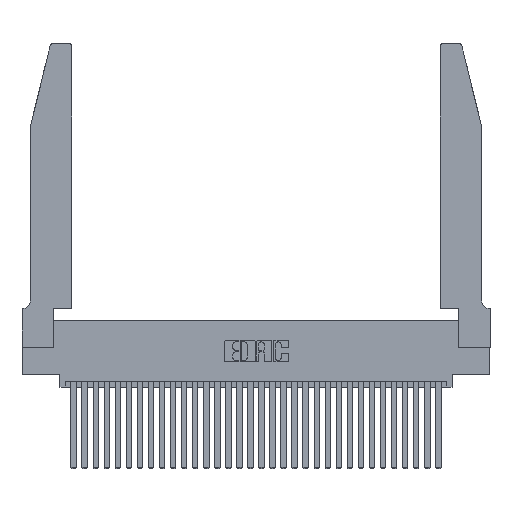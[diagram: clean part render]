
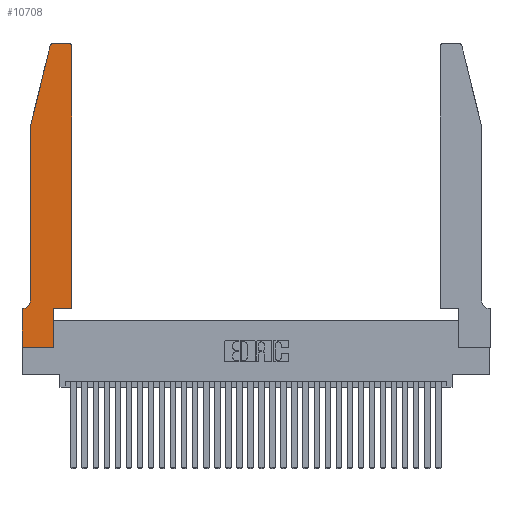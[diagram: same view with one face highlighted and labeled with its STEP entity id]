
A CAD part, top view. The second image highlights one B-rep face of the part: STEP entity #10708.
In plain terms, the highlighted planar face has unit normal (0, 0, 1).
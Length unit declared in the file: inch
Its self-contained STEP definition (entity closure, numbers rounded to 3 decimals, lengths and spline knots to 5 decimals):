
#958 = EDGE_CURVE ( 'NONE', #2977, #4452, #2558, .T. ) ;
#1462 = CARTESIAN_POINT ( 'NONE',  ( 0., 0., 0.37 ) ) ;
#1644 = CARTESIAN_POINT ( 'NONE',  ( 0.284, 2.75, 0.37 ) ) ;
#2005 = CARTESIAN_POINT ( 'NONE',  ( 0.0055, 0.42, 0.37 ) ) ;
#2331 = EDGE_CURVE ( 'NONE', #12128, #19467, #25358, .T. ) ;
#2558 = CIRCLE ( 'NONE', #5105, 0.03 ) ;
#2598 = ORIENTED_EDGE ( 'NONE', *, *, #28789, .T. ) ;
#2977 = VERTEX_POINT ( 'NONE', #1644 ) ;
#3262 = CARTESIAN_POINT ( 'NONE',  ( 0.25487, 2.72718, 0.37 ) ) ;
#3462 = DIRECTION ( 'NONE',  ( 0., 1., 0. ) ) ;
#3615 = CARTESIAN_POINT ( 'NONE',  ( 0.4205, 2.75, 0.37 ) ) ;
#4070 = LINE ( 'NONE', #9349, #22545 ) ;
#4452 = VERTEX_POINT ( 'NONE', #3262 ) ;
#4640 = DIRECTION ( 'NONE',  ( -1., 0., 0. ) ) ;
#5011 = EDGE_LOOP ( 'NONE', ( #26423, #30237, #30179, #9703, #2598, #25439, #15466, #19028, #8001, #28906, #23897, #11461 ) ) ;
#5105 = AXIS2_PLACEMENT_3D ( 'NONE', #8867, #8754, #18470 ) ;
#5704 = DIRECTION ( 'NONE',  ( -0.239, -0.971, 0. ) ) ;
#6570 = CARTESIAN_POINT ( 'NONE',  ( 0.4505, 0.35, 0.37 ) ) ;
#6657 = CARTESIAN_POINT ( 'NONE',  ( 0., 0., 0.37 ) ) ;
#7114 = CARTESIAN_POINT ( 'NONE',  ( 0.4205, 2.72, 0.37 ) ) ;
#7984 = CARTESIAN_POINT ( 'NONE',  ( 0.4505, 0.35, 0.37 ) ) ;
#8001 = ORIENTED_EDGE ( 'NONE', *, *, #20111, .T. ) ;
#8124 = VECTOR ( 'NONE', #22843, 39.37008 ) ;
#8686 = CARTESIAN_POINT ( 'NONE',  ( 0.2865, 0., 0.37 ) ) ;
#8754 = DIRECTION ( 'NONE',  ( 0., 0., 1. ) ) ;
#8867 = CARTESIAN_POINT ( 'NONE',  ( 0.284, 2.72, 0.37 ) ) ;
#8993 = DIRECTION ( 'NONE',  ( 0., 0., 1. ) ) ;
#9085 = LINE ( 'NONE', #15919, #20878 ) ;
#9349 = CARTESIAN_POINT ( 'NONE',  ( 0.0755, 2., 0.37 ) ) ;
#9658 = DIRECTION ( 'NONE',  ( 1., 0., 0. ) ) ;
#9703 = ORIENTED_EDGE ( 'NONE', *, *, #13837, .T. ) ;
#9806 = DIRECTION ( 'NONE',  ( -1., 0., 0. ) ) ;
#9811 = EDGE_CURVE ( 'NONE', #4452, #14387, #9085, .T. ) ;
#9853 = VERTEX_POINT ( 'NONE', #16025 ) ;
#10679 = EDGE_CURVE ( 'NONE', #9853, #25206, #17339, .T. ) ;
#10708 = ADVANCED_FACE ( 'NONE', ( #22335 ), #28796, .T. ) ;
#11073 = CIRCLE ( 'NONE', #18009, 0.07 ) ;
#11461 = ORIENTED_EDGE ( 'NONE', *, *, #2331, .T. ) ;
#11489 = LINE ( 'NONE', #24695, #30460 ) ;
#11821 = EDGE_CURVE ( 'NONE', #19267, #12128, #19568, .T. ) ;
#11926 = CARTESIAN_POINT ( 'NONE',  ( 0., 0.35, 0.37 ) ) ;
#12128 = VERTEX_POINT ( 'NONE', #15202 ) ;
#12404 = CARTESIAN_POINT ( 'NONE',  ( 0.2605, 2.75, 0.37 ) ) ;
#12833 = AXIS2_PLACEMENT_3D ( 'NONE', #7114, #24608, #9658 ) ;
#13027 = LINE ( 'NONE', #1462, #25416 ) ;
#13837 = EDGE_CURVE ( 'NONE', #14387, #19399, #4070, .T. ) ;
#14002 = DIRECTION ( 'NONE',  ( -1., 0., 0. ) ) ;
#14350 = EDGE_CURVE ( 'NONE', #19467, #2977, #30959, .T. ) ;
#14387 = VERTEX_POINT ( 'NONE', #22372 ) ;
#15202 = CARTESIAN_POINT ( 'NONE',  ( 0.4505, 2.72, 0.37 ) ) ;
#15466 = ORIENTED_EDGE ( 'NONE', *, *, #21263, .T. ) ;
#15919 = CARTESIAN_POINT ( 'NONE',  ( 0.0755, 2., 0.37 ) ) ;
#16025 = CARTESIAN_POINT ( 'NONE',  ( 0.0055, 0.35, 0.37 ) ) ;
#16575 = VECTOR ( 'NONE', #14002, 39.37008 ) ;
#16862 = DIRECTION ( 'NONE',  ( 1., 0., 0. ) ) ;
#17339 = LINE ( 'NONE', #21385, #16575 ) ;
#17900 = CARTESIAN_POINT ( 'NONE',  ( 0.4505, 0.35, 0.37 ) ) ;
#18009 = AXIS2_PLACEMENT_3D ( 'NONE', #2005, #19764, #4640 ) ;
#18324 = VECTOR ( 'NONE', #3462, 39.37008 ) ;
#18470 = DIRECTION ( 'NONE',  ( 1., 0., 0. ) ) ;
#19028 = ORIENTED_EDGE ( 'NONE', *, *, #22811, .T. ) ;
#19112 = AXIS2_PLACEMENT_3D ( 'NONE', #21492, #8993, #26432 ) ;
#19267 = VERTEX_POINT ( 'NONE', #7984 ) ;
#19399 = VERTEX_POINT ( 'NONE', #30832 ) ;
#19467 = VERTEX_POINT ( 'NONE', #3615 ) ;
#19568 = LINE ( 'NONE', #6570, #20357 ) ;
#19764 = DIRECTION ( 'NONE',  ( 0., 0., -1. ) ) ;
#20111 = EDGE_CURVE ( 'NONE', #25022, #28366, #24852, .T. ) ;
#20357 = VECTOR ( 'NONE', #24076, 39.37008 ) ;
#20878 = VECTOR ( 'NONE', #5704, 39.37008 ) ;
#21263 = EDGE_CURVE ( 'NONE', #25206, #32402, #11489, .T. ) ;
#21385 = CARTESIAN_POINT ( 'NONE',  ( 0.0755, 0.35, 0.37 ) ) ;
#21492 = CARTESIAN_POINT ( 'NONE',  ( 0., 0.35, 0.37 ) ) ;
#22246 = LINE ( 'NONE', #17900, #8124 ) ;
#22335 = FACE_OUTER_BOUND ( 'NONE', #5011, .T. ) ;
#22372 = CARTESIAN_POINT ( 'NONE',  ( 0.0755, 2., 0.37 ) ) ;
#22545 = VECTOR ( 'NONE', #24403, 39.37008 ) ;
#22811 = EDGE_CURVE ( 'NONE', #32402, #25022, #13027, .T. ) ;
#22843 = DIRECTION ( 'NONE',  ( 1., 0., 0. ) ) ;
#23658 = VECTOR ( 'NONE', #9806, 39.37008 ) ;
#23897 = ORIENTED_EDGE ( 'NONE', *, *, #11821, .T. ) ;
#24076 = DIRECTION ( 'NONE',  ( 0., 1., 0. ) ) ;
#24136 = EDGE_CURVE ( 'NONE', #28366, #19267, #22246, .T. ) ;
#24403 = DIRECTION ( 'NONE',  ( 0., -1., 0. ) ) ;
#24608 = DIRECTION ( 'NONE',  ( 0., 0., 1. ) ) ;
#24695 = CARTESIAN_POINT ( 'NONE',  ( 0., 0., 0.37 ) ) ;
#24852 = LINE ( 'NONE', #25975, #18324 ) ;
#25022 = VERTEX_POINT ( 'NONE', #8686 ) ;
#25206 = VERTEX_POINT ( 'NONE', #11926 ) ;
#25358 = CIRCLE ( 'NONE', #12833, 0.03 ) ;
#25365 = CARTESIAN_POINT ( 'NONE',  ( 0.2865, 0.35, 0.37 ) ) ;
#25416 = VECTOR ( 'NONE', #16862, 39.37008 ) ;
#25439 = ORIENTED_EDGE ( 'NONE', *, *, #10679, .T. ) ;
#25975 = CARTESIAN_POINT ( 'NONE',  ( 0.2865, 0.35, 0.37 ) ) ;
#26423 = ORIENTED_EDGE ( 'NONE', *, *, #14350, .T. ) ;
#26432 = DIRECTION ( 'NONE',  ( 1., 0., 0. ) ) ;
#27377 = DIRECTION ( 'NONE',  ( 0., -1., 0. ) ) ;
#28366 = VERTEX_POINT ( 'NONE', #25365 ) ;
#28789 = EDGE_CURVE ( 'NONE', #19399, #9853, #11073, .T. ) ;
#28796 = PLANE ( 'NONE',  #19112 ) ;
#28906 = ORIENTED_EDGE ( 'NONE', *, *, #24136, .T. ) ;
#30179 = ORIENTED_EDGE ( 'NONE', *, *, #9811, .T. ) ;
#30237 = ORIENTED_EDGE ( 'NONE', *, *, #958, .T. ) ;
#30460 = VECTOR ( 'NONE', #27377, 39.37008 ) ;
#30832 = CARTESIAN_POINT ( 'NONE',  ( 0.0755, 0.42, 0.37 ) ) ;
#30959 = LINE ( 'NONE', #12404, #23658 ) ;
#32402 = VERTEX_POINT ( 'NONE', #6657 ) ;
